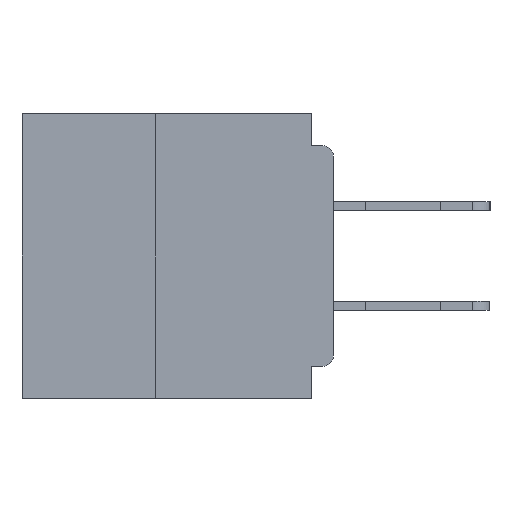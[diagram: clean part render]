
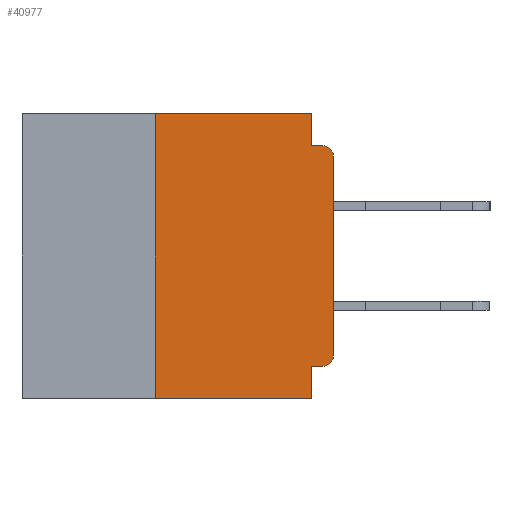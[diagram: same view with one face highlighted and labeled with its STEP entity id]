
A CAD part, left-side view. The second image highlights one B-rep face of the part: STEP entity #40977.
In plain terms, the highlighted planar face has unit normal (-1, 0, 0).
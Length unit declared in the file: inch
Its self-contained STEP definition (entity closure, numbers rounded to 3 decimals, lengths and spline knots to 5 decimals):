
#65 = CARTESIAN_POINT ( 'NONE',  ( 0., 0., -0.355 ) ) ;
#310 = CARTESIAN_POINT ( 'NONE',  ( 0., 0., -0.045 ) ) ;
#458 = LINE ( 'NONE', #9836, #51302 ) ;
#778 = VERTEX_POINT ( 'NONE', #45702 ) ;
#910 = VECTOR ( 'NONE', #7917, 39.37008 ) ;
#1902 = EDGE_CURVE ( 'NONE', #36718, #30401, #458, .T. ) ;
#3080 = PLANE ( 'NONE',  #36016 ) ;
#4454 = DIRECTION ( 'NONE',  ( 0., -1., 0. ) ) ;
#7372 = FACE_OUTER_BOUND ( 'NONE', #22142, .T. ) ;
#7917 = DIRECTION ( 'NONE',  ( 0., 0., 1. ) ) ;
#8195 = CARTESIAN_POINT ( 'NONE',  ( 0., 0.25, -0.4 ) ) ;
#8667 = EDGE_CURVE ( 'NONE', #36718, #38306, #15683, .T. ) ;
#9319 = DIRECTION ( 'NONE',  ( 0., -1., 0. ) ) ;
#9762 = VERTEX_POINT ( 'NONE', #10893 ) ;
#9836 = CARTESIAN_POINT ( 'NONE',  ( 0., 0.437, -0.4 ) ) ;
#9860 = ORIENTED_EDGE ( 'NONE', *, *, #17575, .F. ) ;
#9866 = EDGE_CURVE ( 'NONE', #25493, #30401, #29973, .T. ) ;
#10383 = ORIENTED_EDGE ( 'NONE', *, *, #8667, .F. ) ;
#10893 = CARTESIAN_POINT ( 'NONE',  ( 0., 0.015, -0.045 ) ) ;
#11309 = VECTOR ( 'NONE', #44231, 39.37008 ) ;
#11556 = ORIENTED_EDGE ( 'NONE', *, *, #15283, .T. ) ;
#11673 = EDGE_CURVE ( 'NONE', #13720, #778, #26563, .T. ) ;
#11754 = LINE ( 'NONE', #31915, #910 ) ;
#13720 = VERTEX_POINT ( 'NONE', #27875 ) ;
#15283 = EDGE_CURVE ( 'NONE', #778, #22795, #11754, .T. ) ;
#15683 = LINE ( 'NONE', #8195, #47562 ) ;
#17575 = EDGE_CURVE ( 'NONE', #38306, #40629, #43255, .T. ) ;
#18517 = CARTESIAN_POINT ( 'NONE',  ( 0., 0.25, 0. ) ) ;
#18605 = DIRECTION ( 'NONE',  ( -1., 0., 0. ) ) ;
#18756 = AXIS2_PLACEMENT_3D ( 'NONE', #18932, #46868, #22968 ) ;
#18932 = CARTESIAN_POINT ( 'NONE',  ( 0., 0.015, -0.06 ) ) ;
#20209 = CARTESIAN_POINT ( 'NONE',  ( 0., 0.031, -0.4 ) ) ;
#21944 = LINE ( 'NONE', #24370, #39475 ) ;
#22142 = EDGE_LOOP ( 'NONE', ( #11556, #48466, #37289, #51235, #9860, #10383, #44840, #32020, #38819, #34024 ) ) ;
#22795 = VERTEX_POINT ( 'NONE', #30986 ) ;
#22968 = DIRECTION ( 'NONE',  ( 0., 0., -1. ) ) ;
#23369 = DIRECTION ( 'NONE',  ( 1., 0., 0. ) ) ;
#24291 = DIRECTION ( 'NONE',  ( 0., 1., 0. ) ) ;
#24370 = CARTESIAN_POINT ( 'NONE',  ( 0., 0.031, 0. ) ) ;
#24408 = CIRCLE ( 'NONE', #18756, 0.015 ) ;
#25160 = CARTESIAN_POINT ( 'NONE',  ( 0., 0.031, 0. ) ) ;
#25493 = VERTEX_POINT ( 'NONE', #51819 ) ;
#26563 = CIRCLE ( 'NONE', #36378, 0.015 ) ;
#26738 = CARTESIAN_POINT ( 'NONE',  ( 0., 0.031, -0.045 ) ) ;
#27875 = CARTESIAN_POINT ( 'NONE',  ( 0., 0.015, -0.355 ) ) ;
#28381 = DIRECTION ( 'NONE',  ( 0., 0., -1. ) ) ;
#29714 = EDGE_CURVE ( 'NONE', #40629, #42176, #21944, .T. ) ;
#29973 = LINE ( 'NONE', #20209, #39364 ) ;
#30401 = VERTEX_POINT ( 'NONE', #44546 ) ;
#30986 = CARTESIAN_POINT ( 'NONE',  ( 0., 0., -0.06 ) ) ;
#31632 = EDGE_CURVE ( 'NONE', #13720, #25493, #50415, .T. ) ;
#31915 = CARTESIAN_POINT ( 'NONE',  ( 0., 0., 0. ) ) ;
#32020 = ORIENTED_EDGE ( 'NONE', *, *, #9866, .F. ) ;
#34024 = ORIENTED_EDGE ( 'NONE', *, *, #11673, .T. ) ;
#36016 = AXIS2_PLACEMENT_3D ( 'NONE', #47280, #23369, #51260 ) ;
#36214 = CARTESIAN_POINT ( 'NONE',  ( 0., 0.437, 0. ) ) ;
#36228 = DIRECTION ( 'NONE',  ( 0., 0., 1. ) ) ;
#36378 = AXIS2_PLACEMENT_3D ( 'NONE', #42552, #18605, #46545 ) ;
#36718 = VERTEX_POINT ( 'NONE', #41531 ) ;
#37289 = ORIENTED_EDGE ( 'NONE', *, *, #46820, .F. ) ;
#38306 = VERTEX_POINT ( 'NONE', #18517 ) ;
#38819 = ORIENTED_EDGE ( 'NONE', *, *, #31632, .F. ) ;
#39364 = VECTOR ( 'NONE', #40149, 39.37008 ) ;
#39475 = VECTOR ( 'NONE', #28381, 39.37008 ) ;
#40149 = DIRECTION ( 'NONE',  ( 0., 0., -1. ) ) ;
#40629 = VERTEX_POINT ( 'NONE', #25160 ) ;
#40977 = ADVANCED_FACE ( 'NONE', ( #7372 ), #3080, .F. ) ;
#41128 = VECTOR ( 'NONE', #24291, 39.37008 ) ;
#41531 = CARTESIAN_POINT ( 'NONE',  ( 0., 0.25, -0.4 ) ) ;
#42176 = VERTEX_POINT ( 'NONE', #26738 ) ;
#42552 = CARTESIAN_POINT ( 'NONE',  ( 0., 0.015, -0.34 ) ) ;
#43255 = LINE ( 'NONE', #36214, #11309 ) ;
#44231 = DIRECTION ( 'NONE',  ( 0., -1., 0. ) ) ;
#44546 = CARTESIAN_POINT ( 'NONE',  ( 0., 0.031, -0.4 ) ) ;
#44840 = ORIENTED_EDGE ( 'NONE', *, *, #1902, .T. ) ;
#45702 = CARTESIAN_POINT ( 'NONE',  ( 0., 0., -0.34 ) ) ;
#46124 = LINE ( 'NONE', #310, #47372 ) ;
#46545 = DIRECTION ( 'NONE',  ( 0., 0., -1. ) ) ;
#46570 = EDGE_CURVE ( 'NONE', #22795, #9762, #24408, .T. ) ;
#46820 = EDGE_CURVE ( 'NONE', #42176, #9762, #46124, .T. ) ;
#46868 = DIRECTION ( 'NONE',  ( -1., 0., 0. ) ) ;
#47280 = CARTESIAN_POINT ( 'NONE',  ( 0., 0.437, 0. ) ) ;
#47372 = VECTOR ( 'NONE', #4454, 39.37008 ) ;
#47562 = VECTOR ( 'NONE', #36228, 39.37008 ) ;
#48466 = ORIENTED_EDGE ( 'NONE', *, *, #46570, .T. ) ;
#50415 = LINE ( 'NONE', #65, #41128 ) ;
#51235 = ORIENTED_EDGE ( 'NONE', *, *, #29714, .F. ) ;
#51260 = DIRECTION ( 'NONE',  ( 0., 0., -1. ) ) ;
#51302 = VECTOR ( 'NONE', #9319, 39.37008 ) ;
#51819 = CARTESIAN_POINT ( 'NONE',  ( 0., 0.031, -0.355 ) ) ;
